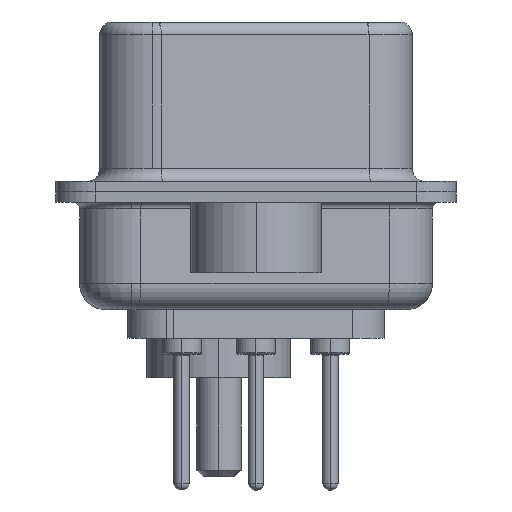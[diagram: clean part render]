
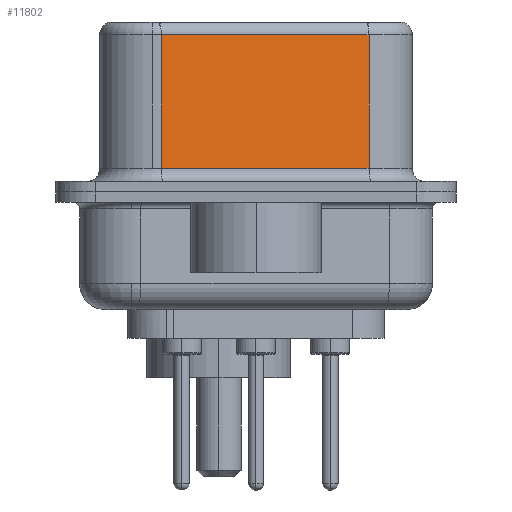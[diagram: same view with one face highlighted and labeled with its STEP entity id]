
A CAD part, left-side view. The second image highlights one B-rep face of the part: STEP entity #11802.
In plain terms, the highlighted planar face has unit normal (-0.985, -0.174, 0).
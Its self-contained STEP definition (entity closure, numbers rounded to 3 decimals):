
#222 = DIRECTION ( 'NONE',  ( -0.174, 0.985, 0. ) ) ;
#1527 = DIRECTION ( 'NONE',  ( 0., 0., -1. ) ) ;
#1845 = FACE_OUTER_BOUND ( 'NONE', #3353, .T. ) ;
#2451 = ORIENTED_EDGE ( 'NONE', *, *, #11039, .T. ) ;
#3101 = AXIS2_PLACEMENT_3D ( 'NONE', #29460, #7303, #222 ) ;
#3353 = EDGE_LOOP ( 'NONE', ( #22565, #22527, #24332, #2451 ) ) ;
#3800 = CARTESIAN_POINT ( 'NONE',  ( 5.132, -4.322, 0.9 ) ) ;
#3928 = CARTESIAN_POINT ( 'NONE',  ( 3.73, 3.628, 6.02 ) ) ;
#5847 = VERTEX_POINT ( 'NONE', #3800 ) ;
#6200 = LINE ( 'NONE', #25220, #25190 ) ;
#6700 = PLANE ( 'NONE',  #3101 ) ;
#7303 = DIRECTION ( 'NONE',  ( 0.985, 0.174, 0. ) ) ;
#7763 = VECTOR ( 'NONE', #28585, 1000. ) ;
#9309 = EDGE_CURVE ( 'NONE', #27018, #5847, #20626, .T. ) ;
#11039 = EDGE_CURVE ( 'NONE', #13030, #5847, #6200, .T. ) ;
#11614 = DIRECTION ( 'NONE',  ( 0.174, -0.985, 0. ) ) ;
#11802 = ADVANCED_FACE ( 'NONE', ( #1845 ), #6700, .F. ) ;
#13030 = VERTEX_POINT ( 'NONE', #24439 ) ;
#13138 = VECTOR ( 'NONE', #21014, 1000. ) ;
#13317 = CARTESIAN_POINT ( 'NONE',  ( 5.132, -4.322, 6.52 ) ) ;
#15116 = EDGE_CURVE ( 'NONE', #24432, #13030, #24998, .T. ) ;
#15238 = VECTOR ( 'NONE', #1527, 1000. ) ;
#17437 = EDGE_CURVE ( 'NONE', #27018, #24432, #19943, .T. ) ;
#18436 = CARTESIAN_POINT ( 'NONE',  ( 5.132, -4.322, 6.02 ) ) ;
#19943 = LINE ( 'NONE', #25809, #13138 ) ;
#20626 = LINE ( 'NONE', #13317, #15238 ) ;
#21014 = DIRECTION ( 'NONE',  ( -0.174, 0.985, 0. ) ) ;
#22527 = ORIENTED_EDGE ( 'NONE', *, *, #17437, .T. ) ;
#22565 = ORIENTED_EDGE ( 'NONE', *, *, #9309, .F. ) ;
#24332 = ORIENTED_EDGE ( 'NONE', *, *, #15116, .T. ) ;
#24432 = VERTEX_POINT ( 'NONE', #3928 ) ;
#24439 = CARTESIAN_POINT ( 'NONE',  ( 3.73, 3.628, 0.9 ) ) ;
#24998 = LINE ( 'NONE', #26605, #7763 ) ;
#25190 = VECTOR ( 'NONE', #11614, 1000. ) ;
#25220 = CARTESIAN_POINT ( 'NONE',  ( 5.132, -4.322, 0.9 ) ) ;
#25809 = CARTESIAN_POINT ( 'NONE',  ( 5.132, -4.322, 6.02 ) ) ;
#26605 = CARTESIAN_POINT ( 'NONE',  ( 3.73, 3.628, 6.52 ) ) ;
#27018 = VERTEX_POINT ( 'NONE', #18436 ) ;
#28585 = DIRECTION ( 'NONE',  ( 0., 0., -1. ) ) ;
#29460 = CARTESIAN_POINT ( 'NONE',  ( 5.132, -4.322, 6.52 ) ) ;
